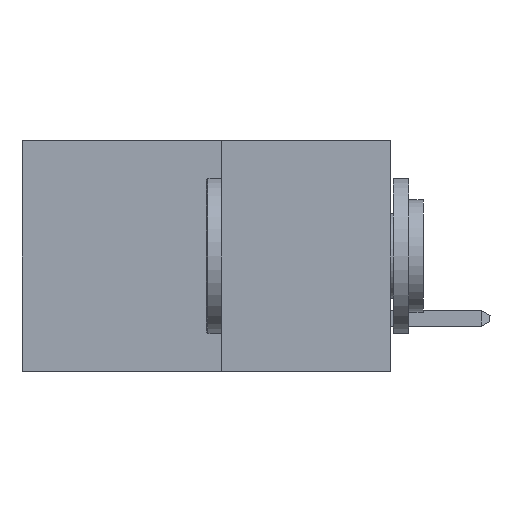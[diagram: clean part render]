
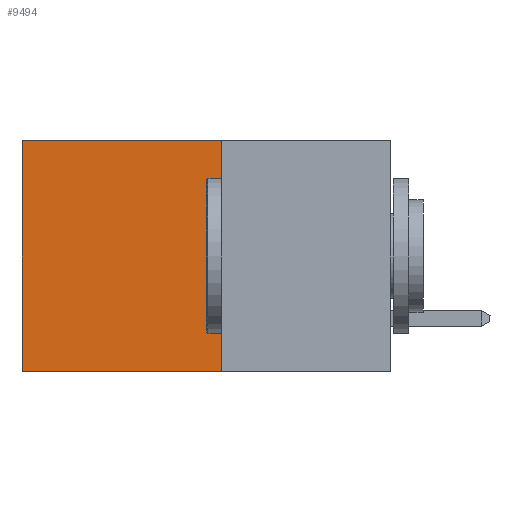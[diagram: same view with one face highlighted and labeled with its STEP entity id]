
A CAD part, left-side view. The second image highlights one B-rep face of the part: STEP entity #9494.
In plain terms, the highlighted planar face has unit normal (-1, 0, 0).
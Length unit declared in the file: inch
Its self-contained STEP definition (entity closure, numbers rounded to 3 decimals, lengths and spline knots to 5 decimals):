
#261 = DIRECTION ( 'NONE',  ( 0., 0., -1. ) ) ;
#525 = ORIENTED_EDGE ( 'NONE', *, *, #13040, .T. ) ;
#537 = VERTEX_POINT ( 'NONE', #11027 ) ;
#904 = CARTESIAN_POINT ( 'NONE',  ( 0.277, 0.27, 0. ) ) ;
#1634 = DIRECTION ( 'NONE',  ( 0., 1., 0. ) ) ;
#2167 = DIRECTION ( 'NONE',  ( 0., 1., 0. ) ) ;
#2430 = VERTEX_POINT ( 'NONE', #14189 ) ;
#2598 = EDGE_CURVE ( 'NONE', #7408, #6756, #5947, .T. ) ;
#2626 = CARTESIAN_POINT ( 'NONE',  ( 0.277, 0.27, -0.37 ) ) ;
#2642 = VECTOR ( 'NONE', #1634, 39.37008 ) ;
#5056 = ORIENTED_EDGE ( 'NONE', *, *, #11789, .T. ) ;
#5375 = DIRECTION ( 'NONE',  ( 0., 0., -1. ) ) ;
#5947 = LINE ( 'NONE', #2626, #2642 ) ;
#6756 = VERTEX_POINT ( 'NONE', #9601 ) ;
#6837 = DIRECTION ( 'NONE',  ( 1., 0., 0. ) ) ;
#7408 = VERTEX_POINT ( 'NONE', #10540 ) ;
#7923 = VECTOR ( 'NONE', #261, 39.37008 ) ;
#8500 = LINE ( 'NONE', #10603, #10926 ) ;
#8901 = ORIENTED_EDGE ( 'NONE', *, *, #2598, .F. ) ;
#9188 = ORIENTED_EDGE ( 'NONE', *, *, #14421, .F. ) ;
#9494 = ADVANCED_FACE ( 'NONE', ( #10173 ), #11933, .F. ) ;
#9601 = CARTESIAN_POINT ( 'NONE',  ( 0.277, 0.59, -0.37 ) ) ;
#10173 = FACE_OUTER_BOUND ( 'NONE', #10451, .T. ) ;
#10451 = EDGE_LOOP ( 'NONE', ( #525, #8901, #9188, #5056 ) ) ;
#10454 = AXIS2_PLACEMENT_3D ( 'NONE', #13062, #6837, #14101 ) ;
#10540 = CARTESIAN_POINT ( 'NONE',  ( 0.277, 0.27, -0.37 ) ) ;
#10603 = CARTESIAN_POINT ( 'NONE',  ( 0.277, 0.59, -0.37 ) ) ;
#10677 = LINE ( 'NONE', #13748, #7923 ) ;
#10926 = VECTOR ( 'NONE', #5375, 39.37008 ) ;
#11027 = CARTESIAN_POINT ( 'NONE',  ( 0.277, 0.27, 0. ) ) ;
#11261 = LINE ( 'NONE', #904, #14066 ) ;
#11789 = EDGE_CURVE ( 'NONE', #537, #2430, #11261, .T. ) ;
#11933 = PLANE ( 'NONE',  #10454 ) ;
#13040 = EDGE_CURVE ( 'NONE', #2430, #6756, #8500, .T. ) ;
#13062 = CARTESIAN_POINT ( 'NONE',  ( 0.277, 0.27, -0.37 ) ) ;
#13748 = CARTESIAN_POINT ( 'NONE',  ( 0.277, 0.27, -0.37 ) ) ;
#14066 = VECTOR ( 'NONE', #2167, 39.37008 ) ;
#14101 = DIRECTION ( 'NONE',  ( 0., 0., -1. ) ) ;
#14189 = CARTESIAN_POINT ( 'NONE',  ( 0.277, 0.59, 0. ) ) ;
#14421 = EDGE_CURVE ( 'NONE', #537, #7408, #10677, .T. ) ;
